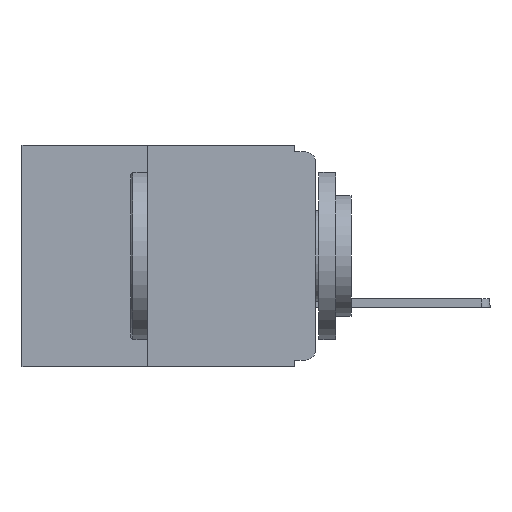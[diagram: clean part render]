
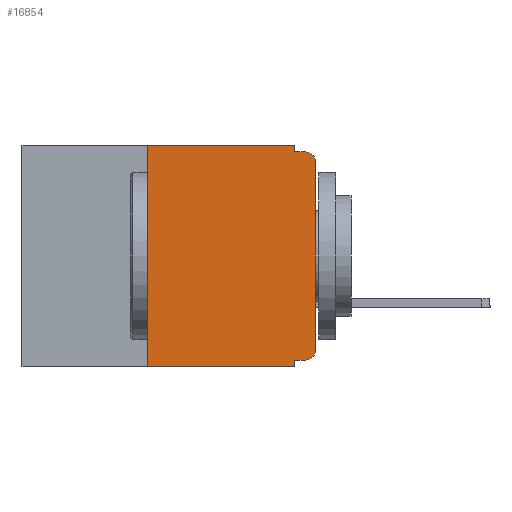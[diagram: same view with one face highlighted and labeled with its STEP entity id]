
A CAD part, left-side view. The second image highlights one B-rep face of the part: STEP entity #16854.
In plain terms, the highlighted planar face has unit normal (-1, 0, 0).
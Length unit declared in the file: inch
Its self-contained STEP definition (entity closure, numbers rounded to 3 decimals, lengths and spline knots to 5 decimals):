
#117 = ORIENTED_EDGE ( 'NONE', *, *, #7097, .F. ) ;
#437 = ORIENTED_EDGE ( 'NONE', *, *, #21784, .F. ) ;
#1795 = ORIENTED_EDGE ( 'NONE', *, *, #22486, .T. ) ;
#2047 = CARTESIAN_POINT ( 'NONE',  ( 0., 0.25, 0. ) ) ;
#2230 = VECTOR ( 'NONE', #14274, 39.37008 ) ;
#2422 = CARTESIAN_POINT ( 'NONE',  ( 0., 0., -0.01 ) ) ;
#2522 = AXIS2_PLACEMENT_3D ( 'NONE', #7742, #25406, #10344 ) ;
#2537 = ORIENTED_EDGE ( 'NONE', *, *, #10019, .T. ) ;
#3972 = VECTOR ( 'NONE', #10716, 39.37008 ) ;
#4175 = VECTOR ( 'NONE', #25566, 39.37008 ) ;
#4234 = ORIENTED_EDGE ( 'NONE', *, *, #27946, .F. ) ;
#5162 = DIRECTION ( 'NONE',  ( 0., 0., -1. ) ) ;
#5326 = VERTEX_POINT ( 'NONE', #32265 ) ;
#5792 = ORIENTED_EDGE ( 'NONE', *, *, #16406, .F. ) ;
#5900 = CARTESIAN_POINT ( 'NONE',  ( 0., 0.437, 0. ) ) ;
#6333 = VECTOR ( 'NONE', #28939, 39.37008 ) ;
#6977 = VERTEX_POINT ( 'NONE', #2047 ) ;
#7097 = EDGE_CURVE ( 'NONE', #5326, #11005, #24422, .T. ) ;
#7742 = CARTESIAN_POINT ( 'NONE',  ( 0., 0.015, -0.025 ) ) ;
#7848 = CIRCLE ( 'NONE', #17229, 0.015 ) ;
#8115 = CARTESIAN_POINT ( 'NONE',  ( 0., 0.437, -0.33 ) ) ;
#8582 = ORIENTED_EDGE ( 'NONE', *, *, #17125, .T. ) ;
#9010 = VECTOR ( 'NONE', #9847, 39.37008 ) ;
#9326 = CARTESIAN_POINT ( 'NONE',  ( 0., 0.437, 0. ) ) ;
#9418 = CARTESIAN_POINT ( 'NONE',  ( 0., 0.015, -0.305 ) ) ;
#9847 = DIRECTION ( 'NONE',  ( 0., 0., 1. ) ) ;
#10019 = EDGE_CURVE ( 'NONE', #24898, #27300, #22846, .T. ) ;
#10344 = DIRECTION ( 'NONE',  ( 0., 0., -1. ) ) ;
#10716 = DIRECTION ( 'NONE',  ( 0., -1., 0. ) ) ;
#10847 = LINE ( 'NONE', #8115, #3972 ) ;
#11005 = VERTEX_POINT ( 'NONE', #22302 ) ;
#11208 = ORIENTED_EDGE ( 'NONE', *, *, #25686, .T. ) ;
#12000 = DIRECTION ( 'NONE',  ( 0., 0., -1. ) ) ;
#12042 = CARTESIAN_POINT ( 'NONE',  ( 0., 0.031, 0. ) ) ;
#12235 = ORIENTED_EDGE ( 'NONE', *, *, #21276, .F. ) ;
#12433 = VECTOR ( 'NONE', #32668, 39.37008 ) ;
#13258 = LINE ( 'NONE', #2422, #12433 ) ;
#13677 = EDGE_CURVE ( 'NONE', #19245, #27300, #13258, .T. ) ;
#13794 = DIRECTION ( 'NONE',  ( 0., 0., -1. ) ) ;
#14274 = DIRECTION ( 'NONE',  ( 0., 1., 0. ) ) ;
#15822 = LINE ( 'NONE', #22319, #9010 ) ;
#15906 = LINE ( 'NONE', #29262, #2230 ) ;
#16406 = EDGE_CURVE ( 'NONE', #6977, #21883, #25245, .T. ) ;
#16854 = ADVANCED_FACE ( 'NONE', ( #30302 ), #28650, .F. ) ;
#17067 = VECTOR ( 'NONE', #29460, 39.37008 ) ;
#17125 = EDGE_CURVE ( 'NONE', #28142, #24898, #15822, .T. ) ;
#17229 = AXIS2_PLACEMENT_3D ( 'NONE', #9418, #27006, #12000 ) ;
#19245 = VERTEX_POINT ( 'NONE', #24727 ) ;
#19307 = VERTEX_POINT ( 'NONE', #24936 ) ;
#21276 = EDGE_CURVE ( 'NONE', #19307, #6977, #32317, .T. ) ;
#21285 = CARTESIAN_POINT ( 'NONE',  ( 0., 0.015, -0.32 ) ) ;
#21784 = EDGE_CURVE ( 'NONE', #26405, #5326, #15906, .T. ) ;
#21883 = VERTEX_POINT ( 'NONE', #12042 ) ;
#22302 = CARTESIAN_POINT ( 'NONE',  ( 0., 0.031, -0.33 ) ) ;
#22319 = CARTESIAN_POINT ( 'NONE',  ( 0., 0., 0. ) ) ;
#22486 = EDGE_CURVE ( 'NONE', #26405, #28142, #7848, .T. ) ;
#22497 = CARTESIAN_POINT ( 'NONE',  ( 0., 0.015, -0.01 ) ) ;
#22846 = CIRCLE ( 'NONE', #2522, 0.015 ) ;
#22895 = CARTESIAN_POINT ( 'NONE',  ( 0., 0.031, 0. ) ) ;
#23231 = ORIENTED_EDGE ( 'NONE', *, *, #13677, .F. ) ;
#24422 = LINE ( 'NONE', #25535, #4175 ) ;
#24727 = CARTESIAN_POINT ( 'NONE',  ( 0., 0.031, -0.01 ) ) ;
#24898 = VERTEX_POINT ( 'NONE', #26690 ) ;
#24936 = CARTESIAN_POINT ( 'NONE',  ( 0., 0.25, -0.33 ) ) ;
#25245 = LINE ( 'NONE', #9326, #17067 ) ;
#25394 = VECTOR ( 'NONE', #5162, 39.37008 ) ;
#25406 = DIRECTION ( 'NONE',  ( -1., 0., 0. ) ) ;
#25535 = CARTESIAN_POINT ( 'NONE',  ( 0., 0.031, -0.33 ) ) ;
#25566 = DIRECTION ( 'NONE',  ( 0., 0., -1. ) ) ;
#25686 = EDGE_CURVE ( 'NONE', #19307, #11005, #10847, .T. ) ;
#26405 = VERTEX_POINT ( 'NONE', #21285 ) ;
#26690 = CARTESIAN_POINT ( 'NONE',  ( 0., 0., -0.025 ) ) ;
#27006 = DIRECTION ( 'NONE',  ( -1., 0., 0. ) ) ;
#27300 = VERTEX_POINT ( 'NONE', #22497 ) ;
#27944 = AXIS2_PLACEMENT_3D ( 'NONE', #5900, #28755, #13794 ) ;
#27946 = EDGE_CURVE ( 'NONE', #21883, #19245, #31992, .T. ) ;
#28142 = VERTEX_POINT ( 'NONE', #31146 ) ;
#28650 = PLANE ( 'NONE',  #27944 ) ;
#28755 = DIRECTION ( 'NONE',  ( 1., 0., 0. ) ) ;
#28939 = DIRECTION ( 'NONE',  ( 0., 0., 1. ) ) ;
#29262 = CARTESIAN_POINT ( 'NONE',  ( 0., 0., -0.32 ) ) ;
#29460 = DIRECTION ( 'NONE',  ( 0., -1., 0. ) ) ;
#30302 = FACE_OUTER_BOUND ( 'NONE', #31914, .T. ) ;
#31146 = CARTESIAN_POINT ( 'NONE',  ( 0., 0., -0.305 ) ) ;
#31530 = CARTESIAN_POINT ( 'NONE',  ( 0., 0.25, -0.33 ) ) ;
#31914 = EDGE_LOOP ( 'NONE', ( #8582, #2537, #23231, #4234, #5792, #12235, #11208, #117, #437, #1795 ) ) ;
#31992 = LINE ( 'NONE', #22895, #25394 ) ;
#32265 = CARTESIAN_POINT ( 'NONE',  ( 0., 0.031, -0.32 ) ) ;
#32317 = LINE ( 'NONE', #31530, #6333 ) ;
#32668 = DIRECTION ( 'NONE',  ( 0., -1., 0. ) ) ;
